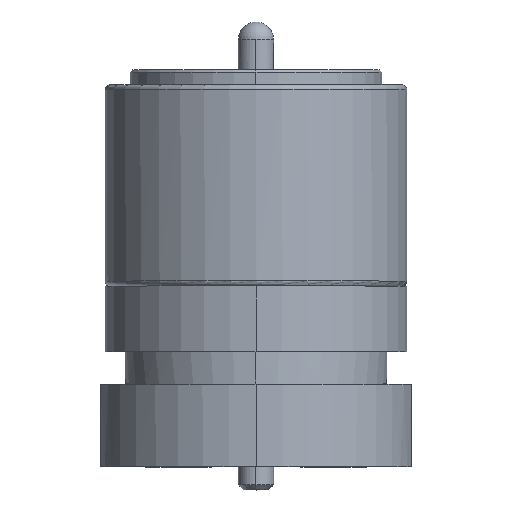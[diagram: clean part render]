
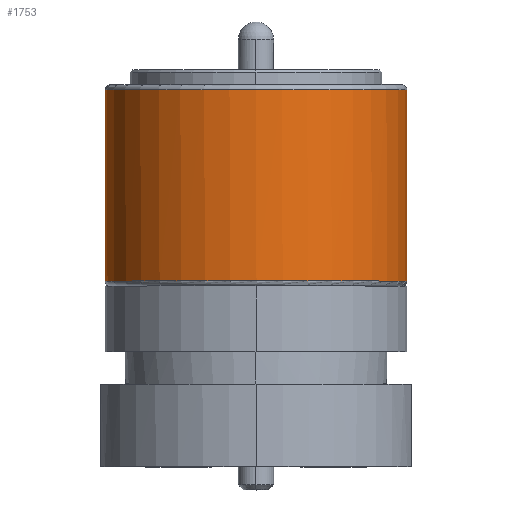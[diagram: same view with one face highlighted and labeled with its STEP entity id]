
A CAD part, top view. The second image highlights one B-rep face of the part: STEP entity #1753.
In plain terms, the highlighted cylindrical face has radius 3 mm (diameter 6 mm), a partial arc.
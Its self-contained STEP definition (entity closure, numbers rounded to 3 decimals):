
#67 = EDGE_CURVE ( 'NONE', #1756, #2709, #1452, .T. ) ;
#78 = CARTESIAN_POINT ( 'NONE',  ( 0., -0.4, 0. ) ) ;
#98 = EDGE_LOOP ( 'NONE', ( #585, #2827, #2866, #447, #1297, #477 ) ) ;
#122 = VERTEX_POINT ( 'NONE', #1287 ) ;
#282 = AXIS2_PLACEMENT_3D ( 'NONE', #417, #1298, #2180 ) ;
#287 = VERTEX_POINT ( 'NONE', #2056 ) ;
#288 = CARTESIAN_POINT ( 'NONE',  ( 0., -4.2, 0. ) ) ;
#324 = CARTESIAN_POINT ( 'NONE',  ( 3., -4.2, 0. ) ) ;
#417 = CARTESIAN_POINT ( 'NONE',  ( 0., -4.276, 0. ) ) ;
#447 = ORIENTED_EDGE ( 'NONE', *, *, #1670, .T. ) ;
#468 = CIRCLE ( 'NONE', #1999, 3. ) ;
#477 = ORIENTED_EDGE ( 'NONE', *, *, #681, .T. ) ;
#480 = EDGE_CURVE ( 'NONE', #514, #122, #2855, .T. ) ;
#514 = VERTEX_POINT ( 'NONE', #2879 ) ;
#517 = DIRECTION ( 'NONE',  ( 0., 1., 0. ) ) ;
#574 = DIRECTION ( 'NONE',  ( 1., 0., 0.005 ) ) ;
#585 = ORIENTED_EDGE ( 'NONE', *, *, #1142, .T. ) ;
#592 = CARTESIAN_POINT ( 'NONE',  ( 3., -0.4, 0.014 ) ) ;
#681 = EDGE_CURVE ( 'NONE', #122, #1782, #2018, .T. ) ;
#692 = CARTESIAN_POINT ( 'NONE',  ( -3., -0.4, 0. ) ) ;
#951 = CARTESIAN_POINT ( 'NONE',  ( 0., -4.2, 0. ) ) ;
#1035 = DIRECTION ( 'NONE',  ( 1., 0., 0. ) ) ;
#1047 = DIRECTION ( 'NONE',  ( 0., -1., 0. ) ) ;
#1060 = AXIS2_PLACEMENT_3D ( 'NONE', #951, #1284, #2611 ) ;
#1075 = CARTESIAN_POINT ( 'NONE',  ( 3., -0.4, 0. ) ) ;
#1105 = CARTESIAN_POINT ( 'NONE',  ( -3., -4.2, 0.02 ) ) ;
#1142 = EDGE_CURVE ( 'NONE', #1782, #287, #1164, .T. ) ;
#1164 = CIRCLE ( 'NONE', #1060, 3. ) ;
#1222 = LINE ( 'NONE', #324, #2555 ) ;
#1284 = DIRECTION ( 'NONE',  ( 0., 1., 0. ) ) ;
#1287 = CARTESIAN_POINT ( 'NONE',  ( -3., -4.2, 0. ) ) ;
#1297 = ORIENTED_EDGE ( 'NONE', *, *, #480, .T. ) ;
#1298 = DIRECTION ( 'NONE',  ( 0., 1., 0. ) ) ;
#1452 = CIRCLE ( 'NONE', #2481, 3. ) ;
#1582 = DIRECTION ( 'NONE',  ( 0., -1., 0. ) ) ;
#1670 = EDGE_CURVE ( 'NONE', #2709, #514, #468, .T. ) ;
#1683 = CARTESIAN_POINT ( 'NONE',  ( 0., -0.4, 0. ) ) ;
#1753 = ADVANCED_FACE ( 'NONE', ( #2632 ), #2402, .T. ) ;
#1756 = VERTEX_POINT ( 'NONE', #1075 ) ;
#1782 = VERTEX_POINT ( 'NONE', #1105 ) ;
#1893 = DIRECTION ( 'NONE',  ( -1., 0., 0. ) ) ;
#1986 = EDGE_CURVE ( 'NONE', #287, #1756, #1222, .T. ) ;
#1999 = AXIS2_PLACEMENT_3D ( 'NONE', #1683, #2569, #574 ) ;
#2018 = CIRCLE ( 'NONE', #2573, 3. ) ;
#2056 = CARTESIAN_POINT ( 'NONE',  ( 3., -4.2, 0. ) ) ;
#2180 = DIRECTION ( 'NONE',  ( -1., 0., 0. ) ) ;
#2402 = CYLINDRICAL_SURFACE ( 'NONE', #282, 3. ) ;
#2481 = AXIS2_PLACEMENT_3D ( 'NONE', #78, #1047, #1035 ) ;
#2555 = VECTOR ( 'NONE', #2580, 1000. ) ;
#2569 = DIRECTION ( 'NONE',  ( 0., -1., 0. ) ) ;
#2573 = AXIS2_PLACEMENT_3D ( 'NONE', #288, #517, #1893 ) ;
#2580 = DIRECTION ( 'NONE',  ( 0., 1., 0. ) ) ;
#2609 = VECTOR ( 'NONE', #1582, 1000. ) ;
#2611 = DIRECTION ( 'NONE',  ( -1., 0., 0.007 ) ) ;
#2632 = FACE_OUTER_BOUND ( 'NONE', #98, .T. ) ;
#2709 = VERTEX_POINT ( 'NONE', #592 ) ;
#2827 = ORIENTED_EDGE ( 'NONE', *, *, #1986, .T. ) ;
#2855 = LINE ( 'NONE', #692, #2609 ) ;
#2866 = ORIENTED_EDGE ( 'NONE', *, *, #67, .T. ) ;
#2879 = CARTESIAN_POINT ( 'NONE',  ( -3., -0.4, 0. ) ) ;
